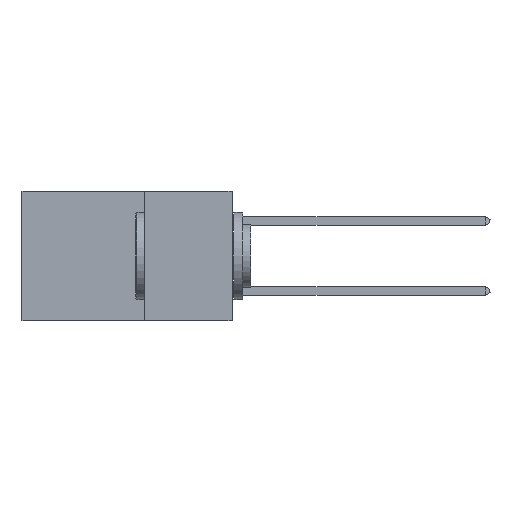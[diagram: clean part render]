
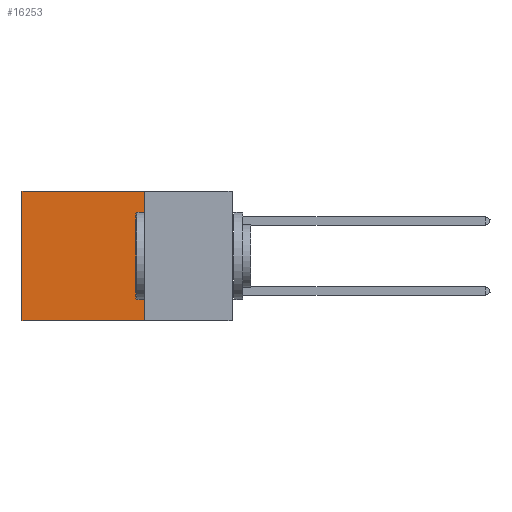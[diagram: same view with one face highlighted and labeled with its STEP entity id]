
A CAD part, left-side view. The second image highlights one B-rep face of the part: STEP entity #16253.
In plain terms, the highlighted planar face has unit normal (-1, 0, 0).
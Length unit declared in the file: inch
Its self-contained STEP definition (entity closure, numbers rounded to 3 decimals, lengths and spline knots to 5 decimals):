
#673 = VERTEX_POINT ( 'NONE', #24450 ) ;
#1083 = EDGE_CURVE ( 'NONE', #673, #18375, #14246, .T. ) ;
#1387 = CARTESIAN_POINT ( 'NONE',  ( 0.2875, 0.25, 0. ) ) ;
#1782 = DIRECTION ( 'NONE',  ( 1., 0., 0. ) ) ;
#2392 = ORIENTED_EDGE ( 'NONE', *, *, #2882, .F. ) ;
#2406 = CARTESIAN_POINT ( 'NONE',  ( 0.2875, 0.25, -0.37 ) ) ;
#2802 = VERTEX_POINT ( 'NONE', #7068 ) ;
#2882 = EDGE_CURVE ( 'NONE', #21957, #18375, #19737, .T. ) ;
#2949 = VECTOR ( 'NONE', #25757, 39.37008 ) ;
#4293 = ORIENTED_EDGE ( 'NONE', *, *, #15059, .F. ) ;
#5762 = DIRECTION ( 'NONE',  ( 0., 0., -1. ) ) ;
#5808 = FACE_OUTER_BOUND ( 'NONE', #18264, .T. ) ;
#6446 = LINE ( 'NONE', #1387, #17672 ) ;
#6628 = CARTESIAN_POINT ( 'NONE',  ( 0.2875, 0.6, -0.37 ) ) ;
#7068 = CARTESIAN_POINT ( 'NONE',  ( 0.2875, 0.25, 0. ) ) ;
#8772 = ORIENTED_EDGE ( 'NONE', *, *, #8936, .T. ) ;
#8936 = EDGE_CURVE ( 'NONE', #2802, #673, #6446, .T. ) ;
#9825 = PLANE ( 'NONE',  #21899 ) ;
#9939 = LINE ( 'NONE', #19676, #25111 ) ;
#11829 = ORIENTED_EDGE ( 'NONE', *, *, #1083, .T. ) ;
#11850 = CARTESIAN_POINT ( 'NONE',  ( 0.2875, 0.25, 0. ) ) ;
#14246 = LINE ( 'NONE', #25793, #2949 ) ;
#15059 = EDGE_CURVE ( 'NONE', #2802, #21957, #9939, .T. ) ;
#15460 = DIRECTION ( 'NONE',  ( 0., 1., 0. ) ) ;
#15832 = DIRECTION ( 'NONE',  ( 0., 0., -1. ) ) ;
#16253 = ADVANCED_FACE ( 'NONE', ( #5808 ), #9825, .F. ) ;
#17255 = DIRECTION ( 'NONE',  ( 0., 1., 0. ) ) ;
#17672 = VECTOR ( 'NONE', #15460, 39.37008 ) ;
#18264 = EDGE_LOOP ( 'NONE', ( #11829, #2392, #4293, #8772 ) ) ;
#18375 = VERTEX_POINT ( 'NONE', #6628 ) ;
#19676 = CARTESIAN_POINT ( 'NONE',  ( 0.2875, 0.25, 0. ) ) ;
#19737 = LINE ( 'NONE', #25070, #24358 ) ;
#21899 = AXIS2_PLACEMENT_3D ( 'NONE', #11850, #1782, #15832 ) ;
#21957 = VERTEX_POINT ( 'NONE', #2406 ) ;
#24358 = VECTOR ( 'NONE', #17255, 39.37008 ) ;
#24450 = CARTESIAN_POINT ( 'NONE',  ( 0.2875, 0.6, 0. ) ) ;
#25070 = CARTESIAN_POINT ( 'NONE',  ( 0.2875, 0.25, -0.37 ) ) ;
#25111 = VECTOR ( 'NONE', #5762, 39.37008 ) ;
#25757 = DIRECTION ( 'NONE',  ( 0., 0., -1. ) ) ;
#25793 = CARTESIAN_POINT ( 'NONE',  ( 0.2875, 0.6, 0. ) ) ;
